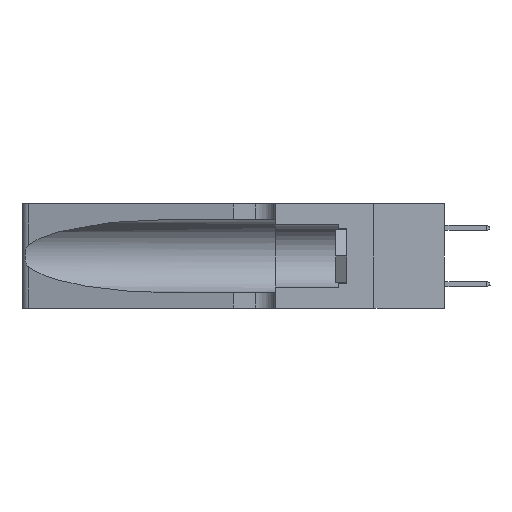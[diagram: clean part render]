
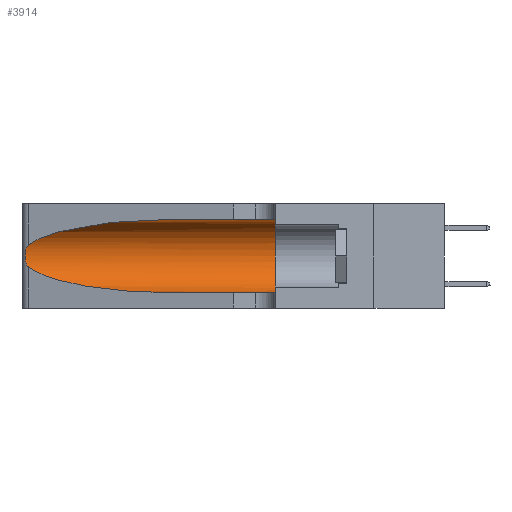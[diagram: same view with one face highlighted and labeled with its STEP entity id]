
A CAD part, left-side view. The second image highlights one B-rep face of the part: STEP entity #3914.
In plain terms, the highlighted cylindrical face has radius 3.308 mm (diameter 6.617 mm), a partial arc.
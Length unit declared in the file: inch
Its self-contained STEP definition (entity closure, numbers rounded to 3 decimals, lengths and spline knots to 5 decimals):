
#158 = VERTEX_POINT ( 'NONE', #22509 ) ;
#782 = CARTESIAN_POINT ( 'NONE',  ( 0.18966, 0.96281, 0.31525 ) ) ;
#854 = CARTESIAN_POINT ( 'NONE',  ( 0.25487, 1.22718, 0.14631 ) ) ;
#1276 = VERTEX_POINT ( 'NONE', #35501 ) ;
#1513 = CARTESIAN_POINT ( 'NONE',  ( 0.1305, 0.35, 0.05475 ) ) ;
#1966 = CARTESIAN_POINT ( 'NONE',  ( 0.1305, 1.61858, 0.185 ) ) ;
#2942 = ORIENTED_EDGE ( 'NONE', *, *, #40475, .T. ) ;
#3215 = DIRECTION ( 'NONE',  ( 0., 1., 0. ) ) ;
#3314 = CYLINDRICAL_SURFACE ( 'NONE', #6983, 0.13025 ) ;
#3914 = ADVANCED_FACE ( 'NONE', ( #41875 ), #3314, .F. ) ;
#4753 =( BOUNDED_CURVE ( )  B_SPLINE_CURVE ( 3, ( #36772, #782, #44193, #8267 ),
 .UNSPECIFIED., .F., .T. ) 
 B_SPLINE_CURVE_WITH_KNOTS ( ( 4, 4 ),
 ( 1.5708, 2.84003 ),
 .UNSPECIFIED. ) 
 CURVE ( )  GEOMETRIC_REPRESENTATION_ITEM ( )  RATIONAL_B_SPLINE_CURVE ( ( 1., 0.87, 0.87, 1. ) ) 
 REPRESENTATION_ITEM ( '' )  );
#5109 = ORIENTED_EDGE ( 'NONE', *, *, #31038, .T. ) ;
#5335 = CARTESIAN_POINT ( 'NONE',  ( 0.25854, 1.2359, 0.20912 ) ) ;
#5355 = B_SPLINE_CURVE_WITH_KNOTS ( 'NONE', 3,
 ( #15981, #27366, #16301, #16612, #5335, #30696, #30547, #34510, #9151, #38144, #37978, #31008, #23275, #37833 ),
 .UNSPECIFIED., .F., .F.,
 ( 4, 2, 2, 2, 2, 2, 4 ),
 ( 0., 0.00027, 0.00053, 0.00107, 0.0016, 0.00187, 0.00214 ),
 .UNSPECIFIED. ) ;
#5648 = VECTOR ( 'NONE', #21332, 39.37008 ) ;
#5874 = ORIENTED_EDGE ( 'NONE', *, *, #46260, .T. ) ;
#6617 = LINE ( 'NONE', #10402, #37807 ) ;
#6983 = AXIS2_PLACEMENT_3D ( 'NONE', #1966, #34490, #34181 ) ;
#7042 = ORIENTED_EDGE ( 'NONE', *, *, #18898, .F. ) ;
#8267 = CARTESIAN_POINT ( 'NONE',  ( 0.25487, 1.22718, 0.22369 ) ) ;
#8476 = CARTESIAN_POINT ( 'NONE',  ( 0.1305, 0.72297, 0.05475 ) ) ;
#9151 = CARTESIAN_POINT ( 'NONE',  ( 0.26017, 1.23833, 0.17102 ) ) ;
#10402 = CARTESIAN_POINT ( 'NONE',  ( 0.1305, 1.61858, 0.05475 ) ) ;
#12226 = CARTESIAN_POINT ( 'NONE',  ( 0.25487, 1.22718, 0.14631 ) ) ;
#14061 = VERTEX_POINT ( 'NONE', #1513 ) ;
#15309 = LINE ( 'NONE', #17996, #5648 ) ;
#15981 = CARTESIAN_POINT ( 'NONE',  ( 0.25487, 1.22718, 0.22369 ) ) ;
#16301 = CARTESIAN_POINT ( 'NONE',  ( 0.25639, 1.23184, 0.21858 ) ) ;
#16612 = CARTESIAN_POINT ( 'NONE',  ( 0.25787, 1.23484, 0.2124 ) ) ;
#17429 = AXIS2_PLACEMENT_3D ( 'NONE', #28579, #3215, #18000 ) ;
#17996 = CARTESIAN_POINT ( 'NONE',  ( 0.1305, 1.61858, 0.31525 ) ) ;
#18000 = DIRECTION ( 'NONE',  ( 0., 0., 1. ) ) ;
#18898 = EDGE_CURVE ( 'NONE', #158, #14061, #39472, .T. ) ;
#20115 = VERTEX_POINT ( 'NONE', #12226 ) ;
#20619 = EDGE_LOOP ( 'NONE', ( #43752, #5109, #5874, #2942, #7042, #35372 ) ) ;
#21332 = DIRECTION ( 'NONE',  ( 0., -1., 0. ) ) ;
#22132 = CARTESIAN_POINT ( 'NONE',  ( 0.1305, 0.72297, 0.31525 ) ) ;
#22509 = CARTESIAN_POINT ( 'NONE',  ( 0.1305, 0.35, 0.31525 ) ) ;
#23275 = CARTESIAN_POINT ( 'NONE',  ( 0.25555, 1.22993, 0.14849 ) ) ;
#24525 =( BOUNDED_CURVE ( )  B_SPLINE_CURVE ( 3, ( #854, #44563, #44095, #8476 ),
 .UNSPECIFIED., .F., .F. ) 
 B_SPLINE_CURVE_WITH_KNOTS ( ( 4, 4 ),
 ( 3.44316, 4.71239 ),
 .UNSPECIFIED. ) 
 CURVE ( )  GEOMETRIC_REPRESENTATION_ITEM ( )  RATIONAL_B_SPLINE_CURVE ( ( 1., 0.87, 0.87, 1. ) ) 
 REPRESENTATION_ITEM ( '' )  );
#26195 = CARTESIAN_POINT ( 'NONE',  ( 0.25487, 1.22718, 0.22369 ) ) ;
#27366 = CARTESIAN_POINT ( 'NONE',  ( 0.25555, 1.22994, 0.2215 ) ) ;
#28579 = CARTESIAN_POINT ( 'NONE',  ( 0.1305, 0.35, 0.185 ) ) ;
#28655 = EDGE_CURVE ( 'NONE', #31431, #158, #15309, .T. ) ;
#30547 = CARTESIAN_POINT ( 'NONE',  ( 0.26075, 1.23896, 0.19203 ) ) ;
#30696 = CARTESIAN_POINT ( 'NONE',  ( 0.26018, 1.23835, 0.19895 ) ) ;
#31008 = CARTESIAN_POINT ( 'NONE',  ( 0.25639, 1.23186, 0.15144 ) ) ;
#31038 = EDGE_CURVE ( 'NONE', #44389, #20115, #5355, .T. ) ;
#31431 = VERTEX_POINT ( 'NONE', #22132 ) ;
#34181 = DIRECTION ( 'NONE',  ( 0., 0., -1. ) ) ;
#34490 = DIRECTION ( 'NONE',  ( 0., -1., 0. ) ) ;
#34510 = CARTESIAN_POINT ( 'NONE',  ( 0.26075, 1.23896, 0.178 ) ) ;
#35372 = ORIENTED_EDGE ( 'NONE', *, *, #28655, .F. ) ;
#35501 = CARTESIAN_POINT ( 'NONE',  ( 0.1305, 0.72297, 0.05475 ) ) ;
#36772 = CARTESIAN_POINT ( 'NONE',  ( 0.1305, 0.72297, 0.31525 ) ) ;
#37807 = VECTOR ( 'NONE', #38914, 39.37008 ) ;
#37833 = CARTESIAN_POINT ( 'NONE',  ( 0.25487, 1.22718, 0.14631 ) ) ;
#37978 = CARTESIAN_POINT ( 'NONE',  ( 0.25789, 1.23486, 0.15765 ) ) ;
#38144 = CARTESIAN_POINT ( 'NONE',  ( 0.25856, 1.23593, 0.16098 ) ) ;
#38914 = DIRECTION ( 'NONE',  ( 0., -1., 0. ) ) ;
#39472 = CIRCLE ( 'NONE', #17429, 0.13025 ) ;
#40475 = EDGE_CURVE ( 'NONE', #1276, #14061, #6617, .T. ) ;
#41875 = FACE_OUTER_BOUND ( 'NONE', #20619, .T. ) ;
#42992 = EDGE_CURVE ( 'NONE', #31431, #44389, #4753, .T. ) ;
#43752 = ORIENTED_EDGE ( 'NONE', *, *, #42992, .T. ) ;
#44095 = CARTESIAN_POINT ( 'NONE',  ( 0.18966, 0.96281, 0.05475 ) ) ;
#44193 = CARTESIAN_POINT ( 'NONE',  ( 0.2373, 1.15595, 0.28018 ) ) ;
#44389 = VERTEX_POINT ( 'NONE', #26195 ) ;
#44563 = CARTESIAN_POINT ( 'NONE',  ( 0.2373, 1.15595, 0.08982 ) ) ;
#46260 = EDGE_CURVE ( 'NONE', #20115, #1276, #24525, .T. ) ;
